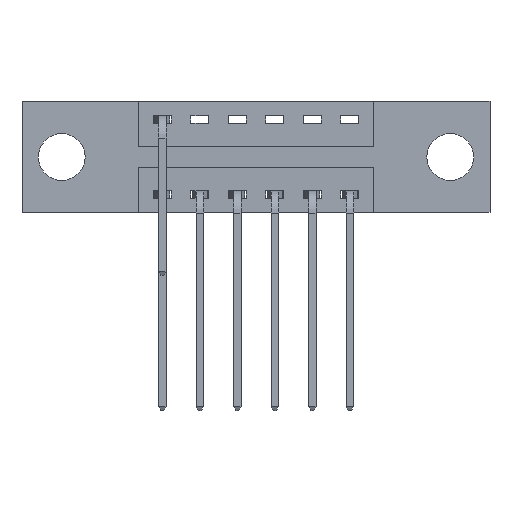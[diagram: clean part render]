
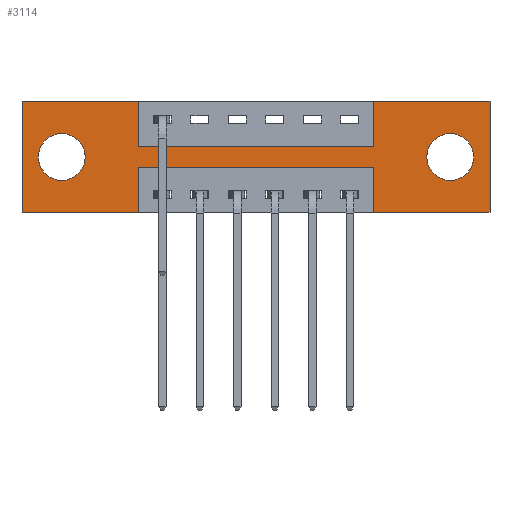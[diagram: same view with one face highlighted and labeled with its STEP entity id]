
A CAD part, front view. The second image highlights one B-rep face of the part: STEP entity #3114.
In plain terms, the highlighted planar face has unit normal (0, -1, 0).
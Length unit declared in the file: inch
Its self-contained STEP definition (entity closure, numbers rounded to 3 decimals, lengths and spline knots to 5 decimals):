
#100 = CIRCLE ( 'NONE', #4872, 0.078 ) ;
#224 = CARTESIAN_POINT ( 'NONE',  ( 0.3875, 0., 0. ) ) ;
#279 = LINE ( 'NONE', #1306, #2253 ) ;
#485 = CARTESIAN_POINT ( 'NONE',  ( 1.1725, 0., -0.22 ) ) ;
#558 = LINE ( 'NONE', #9457, #4977 ) ;
#568 = DIRECTION ( 'NONE',  ( 0., 0., -1. ) ) ;
#840 = ORIENTED_EDGE ( 'NONE', *, *, #6624, .F. ) ;
#879 = VERTEX_POINT ( 'NONE', #8187 ) ;
#971 = VERTEX_POINT ( 'NONE', #1266 ) ;
#1101 = LINE ( 'NONE', #8161, #3359 ) ;
#1140 = ORIENTED_EDGE ( 'NONE', *, *, #8271, .F. ) ;
#1245 = VERTEX_POINT ( 'NONE', #2334 ) ;
#1266 = CARTESIAN_POINT ( 'NONE',  ( 1.1725, 0., -0.15 ) ) ;
#1281 = CARTESIAN_POINT ( 'NONE',  ( 1.4275, 0., -0.263 ) ) ;
#1306 = CARTESIAN_POINT ( 'NONE',  ( 0., 0., -0.37 ) ) ;
#1417 = LINE ( 'NONE', #8441, #9682 ) ;
#1460 = DIRECTION ( 'NONE',  ( -1., 0., 0. ) ) ;
#1705 = CARTESIAN_POINT ( 'NONE',  ( 1.56, 0., 0. ) ) ;
#1725 = EDGE_CURVE ( 'NONE', #6027, #1846, #9845, .T. ) ;
#1846 = VERTEX_POINT ( 'NONE', #3856 ) ;
#1932 = LINE ( 'NONE', #8412, #10370 ) ;
#1969 = AXIS2_PLACEMENT_3D ( 'NONE', #5970, #5941, #10376 ) ;
#2253 = VECTOR ( 'NONE', #3913, 39.37008 ) ;
#2297 = VERTEX_POINT ( 'NONE', #9652 ) ;
#2307 = VERTEX_POINT ( 'NONE', #9535 ) ;
#2334 = CARTESIAN_POINT ( 'NONE',  ( 1.1725, 0., 0. ) ) ;
#2367 = CARTESIAN_POINT ( 'NONE',  ( 0.3875, 0., -0.15 ) ) ;
#2521 = DIRECTION ( 'NONE',  ( 1., 0., 0. ) ) ;
#2603 = DIRECTION ( 'NONE',  ( 0., 1., 0. ) ) ;
#2822 = EDGE_LOOP ( 'NONE', ( #840, #4116, #4903, #3035, #8742, #3687, #1140, #2987, #10210, #3416, #3790, #4324 ) ) ;
#2941 = VERTEX_POINT ( 'NONE', #5780 ) ;
#2987 = ORIENTED_EDGE ( 'NONE', *, *, #3187, .F. ) ;
#3023 = VECTOR ( 'NONE', #7587, 39.37008 ) ;
#3035 = ORIENTED_EDGE ( 'NONE', *, *, #8706, .F. ) ;
#3063 = CARTESIAN_POINT ( 'NONE',  ( 1.56, 0., 0. ) ) ;
#3070 = ORIENTED_EDGE ( 'NONE', *, *, #9243, .T. ) ;
#3088 = LINE ( 'NONE', #5545, #3377 ) ;
#3114 = ADVANCED_FACE ( 'NONE', ( #5803, #9480, #3739 ), #3440, .T. ) ;
#3187 = EDGE_CURVE ( 'NONE', #2941, #971, #6153, .T. ) ;
#3249 = AXIS2_PLACEMENT_3D ( 'NONE', #3461, #3419, #3411 ) ;
#3359 = VECTOR ( 'NONE', #9238, 39.37008 ) ;
#3377 = VECTOR ( 'NONE', #9928, 39.37008 ) ;
#3411 = DIRECTION ( 'NONE',  ( 0., 0., -1. ) ) ;
#3416 = ORIENTED_EDGE ( 'NONE', *, *, #7096, .F. ) ;
#3419 = DIRECTION ( 'NONE',  ( 0., -1., 0. ) ) ;
#3440 = PLANE ( 'NONE',  #3249 ) ;
#3461 = CARTESIAN_POINT ( 'NONE',  ( 0., 0., -0.37 ) ) ;
#3481 = VECTOR ( 'NONE', #9548, 39.37008 ) ;
#3520 = CARTESIAN_POINT ( 'NONE',  ( 1.1725, 0., -0.37 ) ) ;
#3592 = CARTESIAN_POINT ( 'NONE',  ( 0.1325, 0., -0.107 ) ) ;
#3641 = DIRECTION ( 'NONE',  ( 0., 0., -1. ) ) ;
#3686 = CARTESIAN_POINT ( 'NONE',  ( 0.1325, 0., -0.185 ) ) ;
#3687 = ORIENTED_EDGE ( 'NONE', *, *, #4109, .F. ) ;
#3739 = FACE_OUTER_BOUND ( 'NONE', #2822, .T. ) ;
#3790 = ORIENTED_EDGE ( 'NONE', *, *, #6733, .F. ) ;
#3856 = CARTESIAN_POINT ( 'NONE',  ( 1.4275, 0., -0.107 ) ) ;
#3912 = VECTOR ( 'NONE', #568, 39.37008 ) ;
#3913 = DIRECTION ( 'NONE',  ( -1., 0., 0. ) ) ;
#4061 = EDGE_CURVE ( 'NONE', #1846, #6027, #100, .T. ) ;
#4109 = EDGE_CURVE ( 'NONE', #1245, #8266, #7649, .T. ) ;
#4116 = ORIENTED_EDGE ( 'NONE', *, *, #8146, .F. ) ;
#4324 = ORIENTED_EDGE ( 'NONE', *, *, #5147, .F. ) ;
#4558 = VERTEX_POINT ( 'NONE', #10363 ) ;
#4642 = DIRECTION ( 'NONE',  ( 0., 0., 1. ) ) ;
#4872 = AXIS2_PLACEMENT_3D ( 'NONE', #8482, #8459, #8449 ) ;
#4903 = ORIENTED_EDGE ( 'NONE', *, *, #9121, .F. ) ;
#4977 = VECTOR ( 'NONE', #1460, 39.37008 ) ;
#5092 = EDGE_CURVE ( 'NONE', #10026, #2941, #1932, .T. ) ;
#5147 = EDGE_CURVE ( 'NONE', #879, #4558, #1417, .T. ) ;
#5185 = CARTESIAN_POINT ( 'NONE',  ( 0.3875, 0., -0.22 ) ) ;
#5317 = EDGE_LOOP ( 'NONE', ( #3070, #8959 ) ) ;
#5545 = CARTESIAN_POINT ( 'NONE',  ( 0.3875, 0., -0.37 ) ) ;
#5755 = EDGE_LOOP ( 'NONE', ( #7710, #9423 ) ) ;
#5771 = VERTEX_POINT ( 'NONE', #7613 ) ;
#5780 = CARTESIAN_POINT ( 'NONE',  ( 0.3875, 0., -0.15 ) ) ;
#5803 = FACE_BOUND ( 'NONE', #5755, .T. ) ;
#5805 = VERTEX_POINT ( 'NONE', #3592 ) ;
#5837 = LINE ( 'NONE', #6018, #3481 ) ;
#5941 = DIRECTION ( 'NONE',  ( 0., 1., 0. ) ) ;
#5970 = CARTESIAN_POINT ( 'NONE',  ( 1.4275, 0., -0.185 ) ) ;
#6018 = CARTESIAN_POINT ( 'NONE',  ( 1.1725, 0., 0. ) ) ;
#6027 = VERTEX_POINT ( 'NONE', #1281 ) ;
#6153 = LINE ( 'NONE', #2367, #6632 ) ;
#6362 = VERTEX_POINT ( 'NONE', #5185 ) ;
#6506 = CARTESIAN_POINT ( 'NONE',  ( 0.1325, 0., -0.263 ) ) ;
#6624 = EDGE_CURVE ( 'NONE', #6362, #879, #3088, .T. ) ;
#6632 = VECTOR ( 'NONE', #2521, 39.37008 ) ;
#6733 = EDGE_CURVE ( 'NONE', #4558, #2307, #8519, .T. ) ;
#6770 = CIRCLE ( 'NONE', #10397, 0.078 ) ;
#7096 = EDGE_CURVE ( 'NONE', #2307, #10026, #1101, .T. ) ;
#7163 = AXIS2_PLACEMENT_3D ( 'NONE', #7570, #2603, #8295 ) ;
#7167 = CARTESIAN_POINT ( 'NONE',  ( 0., 0., 0. ) ) ;
#7570 = CARTESIAN_POINT ( 'NONE',  ( 0.1325, 0., -0.185 ) ) ;
#7587 = DIRECTION ( 'NONE',  ( 0., 0., 1. ) ) ;
#7613 = CARTESIAN_POINT ( 'NONE',  ( 1.56, 0., -0.37 ) ) ;
#7649 = LINE ( 'NONE', #8123, #7872 ) ;
#7710 = ORIENTED_EDGE ( 'NONE', *, *, #4061, .T. ) ;
#7872 = VECTOR ( 'NONE', #8112, 39.37008 ) ;
#7880 = DIRECTION ( 'NONE',  ( 0., 0., 1. ) ) ;
#8112 = DIRECTION ( 'NONE',  ( 1., 0., 0. ) ) ;
#8123 = CARTESIAN_POINT ( 'NONE',  ( 0., 0., 0. ) ) ;
#8146 = EDGE_CURVE ( 'NONE', #10267, #6362, #558, .T. ) ;
#8161 = CARTESIAN_POINT ( 'NONE',  ( 0., 0., 0. ) ) ;
#8187 = CARTESIAN_POINT ( 'NONE',  ( 0.3875, 0., -0.37 ) ) ;
#8266 = VERTEX_POINT ( 'NONE', #1705 ) ;
#8271 = EDGE_CURVE ( 'NONE', #971, #1245, #5837, .T. ) ;
#8295 = DIRECTION ( 'NONE',  ( 0., 0., 1. ) ) ;
#8318 = EDGE_CURVE ( 'NONE', #9508, #5805, #9288, .T. ) ;
#8412 = CARTESIAN_POINT ( 'NONE',  ( 0.3875, 0., 0. ) ) ;
#8441 = CARTESIAN_POINT ( 'NONE',  ( 0., 0., -0.37 ) ) ;
#8449 = DIRECTION ( 'NONE',  ( 0., 0., -1. ) ) ;
#8459 = DIRECTION ( 'NONE',  ( 0., 1., 0. ) ) ;
#8482 = CARTESIAN_POINT ( 'NONE',  ( 1.4275, 0., -0.185 ) ) ;
#8519 = LINE ( 'NONE', #7167, #8751 ) ;
#8706 = EDGE_CURVE ( 'NONE', #5771, #2297, #279, .T. ) ;
#8742 = ORIENTED_EDGE ( 'NONE', *, *, #9556, .F. ) ;
#8751 = VECTOR ( 'NONE', #7880, 39.37008 ) ;
#8959 = ORIENTED_EDGE ( 'NONE', *, *, #8318, .T. ) ;
#9121 = EDGE_CURVE ( 'NONE', #2297, #10267, #9391, .T. ) ;
#9173 = DIRECTION ( 'NONE',  ( 0., 1., 0. ) ) ;
#9238 = DIRECTION ( 'NONE',  ( 1., 0., 0. ) ) ;
#9243 = EDGE_CURVE ( 'NONE', #5805, #9508, #6770, .T. ) ;
#9288 = CIRCLE ( 'NONE', #7163, 0.078 ) ;
#9391 = LINE ( 'NONE', #3520, #3023 ) ;
#9423 = ORIENTED_EDGE ( 'NONE', *, *, #1725, .T. ) ;
#9457 = CARTESIAN_POINT ( 'NONE',  ( 0.3875, 0., -0.22 ) ) ;
#9480 = FACE_BOUND ( 'NONE', #5317, .T. ) ;
#9508 = VERTEX_POINT ( 'NONE', #6506 ) ;
#9535 = CARTESIAN_POINT ( 'NONE',  ( 0., 0., 0. ) ) ;
#9548 = DIRECTION ( 'NONE',  ( 0., 0., 1. ) ) ;
#9556 = EDGE_CURVE ( 'NONE', #8266, #5771, #10083, .T. ) ;
#9652 = CARTESIAN_POINT ( 'NONE',  ( 1.1725, 0., -0.37 ) ) ;
#9682 = VECTOR ( 'NONE', #9915, 39.37008 ) ;
#9845 = CIRCLE ( 'NONE', #1969, 0.078 ) ;
#9915 = DIRECTION ( 'NONE',  ( -1., 0., 0. ) ) ;
#9928 = DIRECTION ( 'NONE',  ( 0., 0., -1. ) ) ;
#10026 = VERTEX_POINT ( 'NONE', #224 ) ;
#10083 = LINE ( 'NONE', #3063, #3912 ) ;
#10210 = ORIENTED_EDGE ( 'NONE', *, *, #5092, .F. ) ;
#10267 = VERTEX_POINT ( 'NONE', #485 ) ;
#10363 = CARTESIAN_POINT ( 'NONE',  ( 0., 0., -0.37 ) ) ;
#10370 = VECTOR ( 'NONE', #3641, 39.37008 ) ;
#10376 = DIRECTION ( 'NONE',  ( 0., 0., -1. ) ) ;
#10397 = AXIS2_PLACEMENT_3D ( 'NONE', #3686, #9173, #4642 ) ;
